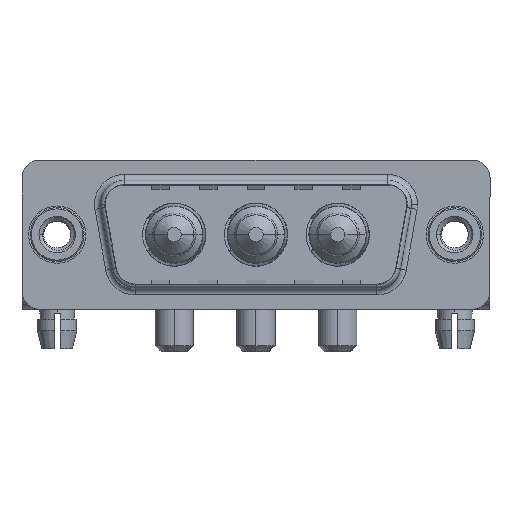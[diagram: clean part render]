
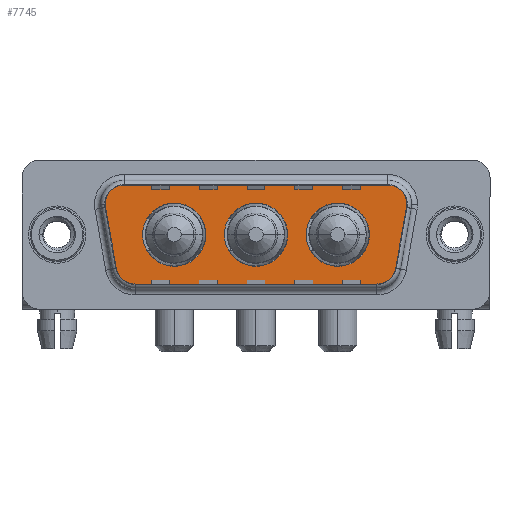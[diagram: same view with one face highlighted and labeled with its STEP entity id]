
A CAD part, top view. The second image highlights one B-rep face of the part: STEP entity #7745.
In plain terms, the highlighted planar face has unit normal (0, 0, 1).
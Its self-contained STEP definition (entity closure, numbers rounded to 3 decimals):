
#47 = DIRECTION ( 'NONE',  ( -1., 0., 0. ) ) ;
#143 = EDGE_CURVE ( 'NONE', #3210, #14279, #961, .T. ) ;
#309 = VECTOR ( 'NONE', #7423, 1000. ) ;
#427 = CARTESIAN_POINT ( 'NONE',  ( 23.5, 0., 0. ) ) ;
#606 = ORIENTED_EDGE ( 'NONE', *, *, #2344, .F. ) ;
#656 = CARTESIAN_POINT ( 'NONE',  ( 5.411, 4.9, 0. ) ) ;
#674 = ORIENTED_EDGE ( 'NONE', *, *, #1059, .F. ) ;
#716 = DIRECTION ( 'NONE',  ( 0., 0., 1. ) ) ;
#730 = VERTEX_POINT ( 'NONE', #3520 ) ;
#961 = LINE ( 'NONE', #12230, #1038 ) ;
#1038 = VECTOR ( 'NONE', #3368, 1000. ) ;
#1059 = EDGE_CURVE ( 'NONE', #13380, #5479, #11954, .T. ) ;
#1071 = EDGE_CURVE ( 'NONE', #14496, #11668, #14354, .T. ) ;
#1149 = EDGE_LOOP ( 'NONE', ( #9172, #606 ) ) ;
#1643 = AXIS2_PLACEMENT_3D ( 'NONE', #1999, #8391, #7134 ) ;
#1680 = CARTESIAN_POINT ( 'NONE',  ( 4.464, -3.247, 0. ) ) ;
#1765 = CARTESIAN_POINT ( 'NONE',  ( 28.836, -3.247, 0. ) ) ;
#1906 = VERTEX_POINT ( 'NONE', #12127 ) ;
#1999 = CARTESIAN_POINT ( 'NONE',  ( 16.65, 0., 0. ) ) ;
#2067 = DIRECTION ( 'NONE',  ( 0., 0., 1. ) ) ;
#2199 = VERTEX_POINT ( 'NONE', #1765 ) ;
#2223 = CARTESIAN_POINT ( 'NONE',  ( 5.411, 2.9, 0. ) ) ;
#2271 = AXIS2_PLACEMENT_3D ( 'NONE', #7756, #15237, #13734 ) ;
#2344 = EDGE_CURVE ( 'NONE', #730, #12077, #2525, .T. ) ;
#2473 = ORIENTED_EDGE ( 'NONE', *, *, #4350, .T. ) ;
#2525 = CIRCLE ( 'NONE', #11784, 2.65 ) ;
#2621 = DIRECTION ( 'NONE',  ( 0., 0., 1. ) ) ;
#2696 = CARTESIAN_POINT ( 'NONE',  ( 26.866, -4.9, 0. ) ) ;
#2809 = DIRECTION ( 'NONE',  ( 0., 0., 1. ) ) ;
#3047 = DIRECTION ( 'NONE',  ( -1., 0., 0. ) ) ;
#3060 = AXIS2_PLACEMENT_3D ( 'NONE', #12733, #5194, #47 ) ;
#3079 = CARTESIAN_POINT ( 'NONE',  ( 3.441, 2.553, 0. ) ) ;
#3210 = VERTEX_POINT ( 'NONE', #14089 ) ;
#3368 = DIRECTION ( 'NONE',  ( 1., 0., 0. ) ) ;
#3389 = DIRECTION ( 'NONE',  ( 0., 0., 1. ) ) ;
#3520 = CARTESIAN_POINT ( 'NONE',  ( 20.85, 0., 0. ) ) ;
#3763 = CIRCLE ( 'NONE', #15415, 2.65 ) ;
#3791 = FACE_BOUND ( 'NONE', #9150, .T. ) ;
#4347 = ORIENTED_EDGE ( 'NONE', *, *, #4923, .T. ) ;
#4350 = EDGE_CURVE ( 'NONE', #11668, #10910, #13262, .T. ) ;
#4394 = DIRECTION ( 'NONE',  ( -1., 0., 0. ) ) ;
#4407 = AXIS2_PLACEMENT_3D ( 'NONE', #4624, #3389, #7199 ) ;
#4551 = CARTESIAN_POINT ( 'NONE',  ( 5.411, 4.9, 0. ) ) ;
#4624 = CARTESIAN_POINT ( 'NONE',  ( 23.5, 0., 0. ) ) ;
#4645 = CIRCLE ( 'NONE', #3060, 2. ) ;
#4808 = DIRECTION ( 'NONE',  ( 1., 0., 0. ) ) ;
#4912 = CIRCLE ( 'NONE', #2271, 2.65 ) ;
#4923 = EDGE_CURVE ( 'NONE', #10910, #14960, #10865, .T. ) ;
#5188 = CARTESIAN_POINT ( 'NONE',  ( 29.859, 2.553, 0. ) ) ;
#5194 = DIRECTION ( 'NONE',  ( 0., 0., 1. ) ) ;
#5479 = VERTEX_POINT ( 'NONE', #7394 ) ;
#5690 = VERTEX_POINT ( 'NONE', #13438 ) ;
#5851 = EDGE_CURVE ( 'NONE', #1906, #5690, #3763, .T. ) ;
#5871 = VECTOR ( 'NONE', #7508, 1000. ) ;
#5895 = DIRECTION ( 'NONE',  ( 1., 0., 0. ) ) ;
#5922 = CIRCLE ( 'NONE', #6711, 2. ) ;
#6259 = CARTESIAN_POINT ( 'NONE',  ( 26.866, -2.9, 0. ) ) ;
#6711 = AXIS2_PLACEMENT_3D ( 'NONE', #10411, #11746, #14324 ) ;
#7134 = DIRECTION ( 'NONE',  ( 1., 0., 0. ) ) ;
#7199 = DIRECTION ( 'NONE',  ( 1., 0., 0. ) ) ;
#7374 = DIRECTION ( 'NONE',  ( 0., 0., 1. ) ) ;
#7394 = CARTESIAN_POINT ( 'NONE',  ( 14., 0., 0. ) ) ;
#7423 = DIRECTION ( 'NONE',  ( 0.174, 0.985, 0. ) ) ;
#7429 = AXIS2_PLACEMENT_3D ( 'NONE', #2223, #716, #13744 ) ;
#7508 = DIRECTION ( 'NONE',  ( 0.174, -0.985, 0. ) ) ;
#7635 = ORIENTED_EDGE ( 'NONE', *, *, #11582, .F. ) ;
#7661 = EDGE_CURVE ( 'NONE', #2199, #11717, #12481, .T. ) ;
#7716 = EDGE_CURVE ( 'NONE', #14960, #8014, #16318, .T. ) ;
#7745 = ADVANCED_FACE ( 'NONE', ( #3791, #10081, #10233, #12562 ), #14060, .T. ) ;
#7756 = CARTESIAN_POINT ( 'NONE',  ( 16.65, 0., 0. ) ) ;
#8014 = VERTEX_POINT ( 'NONE', #1680 ) ;
#8151 = ORIENTED_EDGE ( 'NONE', *, *, #11367, .T. ) ;
#8216 = DIRECTION ( 'NONE',  ( 0., 0., 1. ) ) ;
#8391 = DIRECTION ( 'NONE',  ( 0., 0., 1. ) ) ;
#8626 = AXIS2_PLACEMENT_3D ( 'NONE', #15663, #2809, #3047 ) ;
#9150 = EDGE_LOOP ( 'NONE', ( #674, #7635 ) ) ;
#9170 = CIRCLE ( 'NONE', #16031, 2.65 ) ;
#9172 = ORIENTED_EDGE ( 'NONE', *, *, #14161, .F. ) ;
#9741 = ORIENTED_EDGE ( 'NONE', *, *, #7661, .T. ) ;
#9924 = EDGE_CURVE ( 'NONE', #14279, #2199, #5922, .T. ) ;
#10070 = EDGE_LOOP ( 'NONE', ( #14402, #15567 ) ) ;
#10081 = FACE_BOUND ( 'NONE', #1149, .T. ) ;
#10090 = ORIENTED_EDGE ( 'NONE', *, *, #1071, .T. ) ;
#10233 = FACE_BOUND ( 'NONE', #10070, .T. ) ;
#10411 = CARTESIAN_POINT ( 'NONE',  ( 26.866, -2.9, 0. ) ) ;
#10540 = DIRECTION ( 'NONE',  ( 0., 0., 1. ) ) ;
#10718 = CIRCLE ( 'NONE', #8626, 2. ) ;
#10865 = CIRCLE ( 'NONE', #7429, 2. ) ;
#10910 = VERTEX_POINT ( 'NONE', #4551 ) ;
#11016 = CARTESIAN_POINT ( 'NONE',  ( 9.8, 0., 0. ) ) ;
#11367 = EDGE_CURVE ( 'NONE', #8014, #3210, #10718, .T. ) ;
#11393 = CARTESIAN_POINT ( 'NONE',  ( 29.859, 2.553, 0. ) ) ;
#11548 = CIRCLE ( 'NONE', #4407, 2.65 ) ;
#11582 = EDGE_CURVE ( 'NONE', #5479, #13380, #4912, .T. ) ;
#11668 = VERTEX_POINT ( 'NONE', #13904 ) ;
#11717 = VERTEX_POINT ( 'NONE', #5188 ) ;
#11746 = DIRECTION ( 'NONE',  ( 0., 0., 1. ) ) ;
#11784 = AXIS2_PLACEMENT_3D ( 'NONE', #427, #10540, #5895 ) ;
#11954 = CIRCLE ( 'NONE', #1643, 2.65 ) ;
#12077 = VERTEX_POINT ( 'NONE', #13636 ) ;
#12127 = CARTESIAN_POINT ( 'NONE',  ( 12.45, 0., 0. ) ) ;
#12220 = CARTESIAN_POINT ( 'NONE',  ( 19.3, 0., 0. ) ) ;
#12230 = CARTESIAN_POINT ( 'NONE',  ( 6.434, -4.9, 0. ) ) ;
#12481 = LINE ( 'NONE', #11393, #309 ) ;
#12506 = AXIS2_PLACEMENT_3D ( 'NONE', #13184, #8216, #13271 ) ;
#12507 = EDGE_CURVE ( 'NONE', #5690, #1906, #9170, .T. ) ;
#12562 = FACE_OUTER_BOUND ( 'NONE', #16324, .T. ) ;
#12642 = DIRECTION ( 'NONE',  ( 1., 0., 0. ) ) ;
#12733 = CARTESIAN_POINT ( 'NONE',  ( 27.889, 2.9, 0. ) ) ;
#12981 = EDGE_CURVE ( 'NONE', #11717, #14496, #4645, .T. ) ;
#13184 = CARTESIAN_POINT ( 'NONE',  ( 27.889, 2.9, 0. ) ) ;
#13262 = LINE ( 'NONE', #656, #13781 ) ;
#13271 = DIRECTION ( 'NONE',  ( -1., 0., 0. ) ) ;
#13380 = VERTEX_POINT ( 'NONE', #12220 ) ;
#13438 = CARTESIAN_POINT ( 'NONE',  ( 7.15, 0., 0. ) ) ;
#13456 = CARTESIAN_POINT ( 'NONE',  ( 29.889, 2.9, 0. ) ) ;
#13636 = CARTESIAN_POINT ( 'NONE',  ( 26.15, 0., 0. ) ) ;
#13734 = DIRECTION ( 'NONE',  ( 1., 0., 0. ) ) ;
#13744 = DIRECTION ( 'NONE',  ( 1., 0., 0. ) ) ;
#13759 = DIRECTION ( 'NONE',  ( 1., 0., 0. ) ) ;
#13781 = VECTOR ( 'NONE', #4394, 1000. ) ;
#13904 = CARTESIAN_POINT ( 'NONE',  ( 27.889, 4.9, 0. ) ) ;
#13992 = ORIENTED_EDGE ( 'NONE', *, *, #9924, .T. ) ;
#14060 = PLANE ( 'NONE',  #16216 ) ;
#14089 = CARTESIAN_POINT ( 'NONE',  ( 6.434, -4.9, 0. ) ) ;
#14161 = EDGE_CURVE ( 'NONE', #12077, #730, #11548, .T. ) ;
#14279 = VERTEX_POINT ( 'NONE', #2696 ) ;
#14324 = DIRECTION ( 'NONE',  ( 1., 0., 0. ) ) ;
#14354 = CIRCLE ( 'NONE', #12506, 2. ) ;
#14402 = ORIENTED_EDGE ( 'NONE', *, *, #5851, .F. ) ;
#14496 = VERTEX_POINT ( 'NONE', #13456 ) ;
#14960 = VERTEX_POINT ( 'NONE', #3079 ) ;
#15235 = CARTESIAN_POINT ( 'NONE',  ( 3.441, 2.553, 0. ) ) ;
#15237 = DIRECTION ( 'NONE',  ( 0., 0., 1. ) ) ;
#15415 = AXIS2_PLACEMENT_3D ( 'NONE', #11016, #7374, #4808 ) ;
#15567 = ORIENTED_EDGE ( 'NONE', *, *, #12507, .F. ) ;
#15663 = CARTESIAN_POINT ( 'NONE',  ( 6.434, -2.9, 0. ) ) ;
#15944 = ORIENTED_EDGE ( 'NONE', *, *, #12981, .T. ) ;
#16006 = ORIENTED_EDGE ( 'NONE', *, *, #7716, .T. ) ;
#16031 = AXIS2_PLACEMENT_3D ( 'NONE', #16175, #2067, #13759 ) ;
#16175 = CARTESIAN_POINT ( 'NONE',  ( 9.8, 0., 0. ) ) ;
#16216 = AXIS2_PLACEMENT_3D ( 'NONE', #6259, #2621, #12642 ) ;
#16318 = LINE ( 'NONE', #15235, #5871 ) ;
#16324 = EDGE_LOOP ( 'NONE', ( #13992, #9741, #15944, #10090, #2473, #4347, #16006, #8151, #16422 ) ) ;
#16422 = ORIENTED_EDGE ( 'NONE', *, *, #143, .T. ) ;
